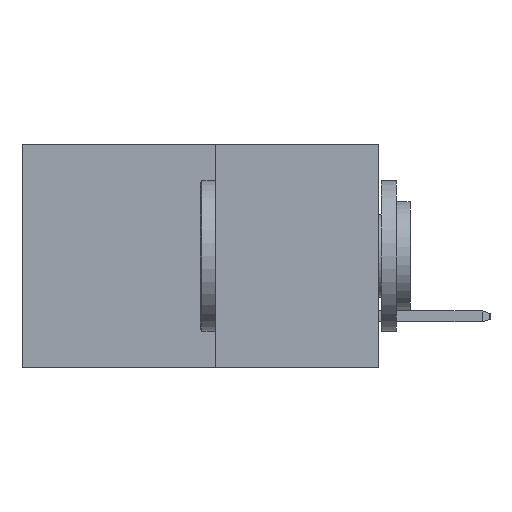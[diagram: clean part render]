
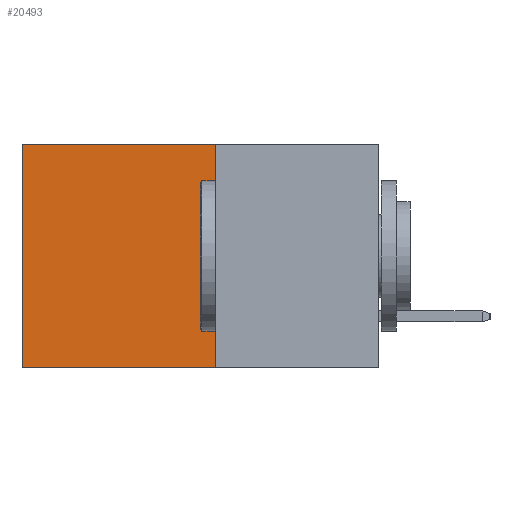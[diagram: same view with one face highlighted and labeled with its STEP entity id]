
A CAD part, left-side view. The second image highlights one B-rep face of the part: STEP entity #20493.
In plain terms, the highlighted planar face has unit normal (-1, 0, 0).
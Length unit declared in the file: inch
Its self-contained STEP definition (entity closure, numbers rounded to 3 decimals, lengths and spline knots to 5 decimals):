
#686 = CARTESIAN_POINT ( 'NONE',  ( 0.277, 0.27, -0.37 ) ) ;
#893 = ORIENTED_EDGE ( 'NONE', *, *, #26639, .T. ) ;
#1713 = EDGE_CURVE ( 'NONE', #5647, #7549, #13645, .T. ) ;
#2551 = ORIENTED_EDGE ( 'NONE', *, *, #1713, .T. ) ;
#3615 = CARTESIAN_POINT ( 'NONE',  ( 0.277, 0.59, -0.37 ) ) ;
#3668 = VECTOR ( 'NONE', #20729, 39.37008 ) ;
#3996 = CARTESIAN_POINT ( 'NONE',  ( 0.277, 0.59, 0. ) ) ;
#4485 = LINE ( 'NONE', #18084, #9839 ) ;
#5647 = VERTEX_POINT ( 'NONE', #3996 ) ;
#6239 = ORIENTED_EDGE ( 'NONE', *, *, #19504, .F. ) ;
#7188 = VERTEX_POINT ( 'NONE', #10730 ) ;
#7549 = VERTEX_POINT ( 'NONE', #20835 ) ;
#9388 = DIRECTION ( 'NONE',  ( 1., 0., 0. ) ) ;
#9668 = VECTOR ( 'NONE', #19069, 39.37008 ) ;
#9839 = VECTOR ( 'NONE', #11544, 39.37008 ) ;
#10362 = FACE_OUTER_BOUND ( 'NONE', #21634, .T. ) ;
#10436 = CARTESIAN_POINT ( 'NONE',  ( 0.277, 0.27, -0.37 ) ) ;
#10730 = CARTESIAN_POINT ( 'NONE',  ( 0.277, 0.27, -0.37 ) ) ;
#11544 = DIRECTION ( 'NONE',  ( 0., 1., 0. ) ) ;
#13645 = LINE ( 'NONE', #3615, #18704 ) ;
#13727 = VERTEX_POINT ( 'NONE', #16772 ) ;
#13735 = PLANE ( 'NONE',  #21041 ) ;
#13834 = ORIENTED_EDGE ( 'NONE', *, *, #18266, .F. ) ;
#16772 = CARTESIAN_POINT ( 'NONE',  ( 0.277, 0.27, 0. ) ) ;
#18084 = CARTESIAN_POINT ( 'NONE',  ( 0.277, 0.27, 0. ) ) ;
#18266 = EDGE_CURVE ( 'NONE', #7188, #7549, #21324, .T. ) ;
#18704 = VECTOR ( 'NONE', #26268, 39.37008 ) ;
#19069 = DIRECTION ( 'NONE',  ( 0., 0., -1. ) ) ;
#19504 = EDGE_CURVE ( 'NONE', #13727, #7188, #25720, .T. ) ;
#20493 = ADVANCED_FACE ( 'NONE', ( #10362 ), #13735, .F. ) ;
#20729 = DIRECTION ( 'NONE',  ( 0., 1., 0. ) ) ;
#20835 = CARTESIAN_POINT ( 'NONE',  ( 0.277, 0.59, -0.37 ) ) ;
#21041 = AXIS2_PLACEMENT_3D ( 'NONE', #22468, #9388, #24657 ) ;
#21324 = LINE ( 'NONE', #686, #3668 ) ;
#21634 = EDGE_LOOP ( 'NONE', ( #2551, #13834, #6239, #893 ) ) ;
#22468 = CARTESIAN_POINT ( 'NONE',  ( 0.277, 0.27, -0.37 ) ) ;
#24657 = DIRECTION ( 'NONE',  ( 0., 0., -1. ) ) ;
#25720 = LINE ( 'NONE', #10436, #9668 ) ;
#26268 = DIRECTION ( 'NONE',  ( 0., 0., -1. ) ) ;
#26639 = EDGE_CURVE ( 'NONE', #13727, #5647, #4485, .T. ) ;
